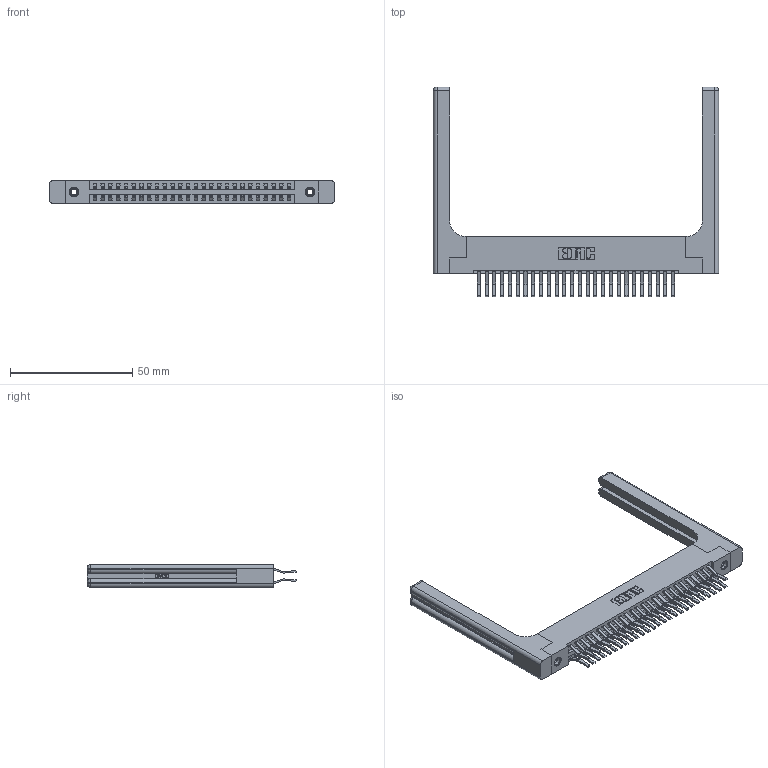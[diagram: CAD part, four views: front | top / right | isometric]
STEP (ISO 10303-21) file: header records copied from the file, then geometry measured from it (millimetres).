
FILE_DESCRIPTION (( 'STEP AP203' ), '1' );
FILE_NAME ('396-052-560-258.STEP', '2019-10-30T13:57:01', ( '' ), ( '' ), 'SwSTEP 2.0', 'SolidWorks 2016', '' );
FILE_SCHEMA (( 'CONFIG_CONTROL_DESIGN' ));
Length unit declared in the file: inch
Products named in the file (5): 345-250-001_345-250-001-102; 346 Part_Flush Mounting Lugs - 0.156 Dia-TH; 396-052-560-258; 345-292-001_560 Tail; 346-220-058_345-220-058
Assembly tree (57 placements, depth 2):
  396-052-560-258
    346 Part_Flush Mounting Lugs - 0.156 Dia-TH
    345-292-001_560 Tail  x52
    345-250-001_345-250-001-102  x2
    346-220-058_345-220-058  x2
Bounding box: 116.61 x 85.74 x 9.4 mm (x, y, z)
Volume: 19081.9 mm3; surface area: 21558.6 mm2
Topology: 57 solids, 57 shells, 3186 faces, 9367 edges, 6154 vertices
Faces by surface type: plane 2044, cylinder 1082, bspline 36, cone 12, sphere 8, torus 4
Entity records: 24392 total; most frequent: CARTESIAN_POINT 5049, ORIENTED_EDGE 3780, DIRECTION 3438, EDGE_CURVE 1890, LINE 1558, VECTOR 1558, VERTEX_POINT 1250, AXIS2_PLACEMENT_3D 940
